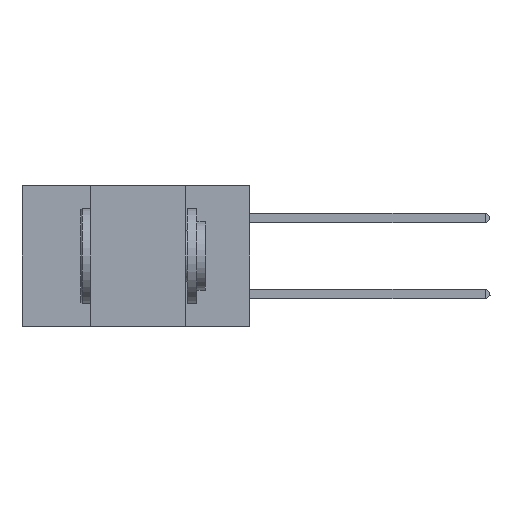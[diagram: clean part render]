
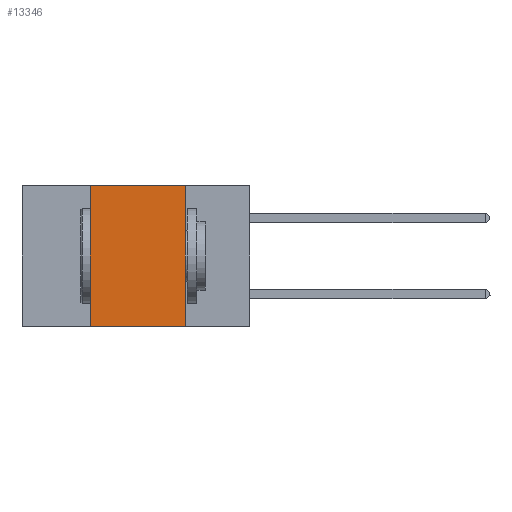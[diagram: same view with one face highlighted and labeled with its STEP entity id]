
A CAD part, left-side view. The second image highlights one B-rep face of the part: STEP entity #13346.
In plain terms, the highlighted planar face has unit normal (-1, 0, 0).
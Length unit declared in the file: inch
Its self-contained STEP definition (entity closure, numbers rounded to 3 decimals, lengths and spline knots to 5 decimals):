
#1140 = CARTESIAN_POINT ( 'NONE',  ( 0., 0.6, -0.37 ) ) ;
#1957 = DIRECTION ( 'NONE',  ( 1., 0., 0. ) ) ;
#2320 = ORIENTED_EDGE ( 'NONE', *, *, #23220, .F. ) ;
#3202 = CARTESIAN_POINT ( 'NONE',  ( 0., 0.42, 0. ) ) ;
#3345 = DIRECTION ( 'NONE',  ( 0., -1., 0. ) ) ;
#3519 = DIRECTION ( 'NONE',  ( 0., 0., -1. ) ) ;
#6569 = ORIENTED_EDGE ( 'NONE', *, *, #11300, .F. ) ;
#9484 = CARTESIAN_POINT ( 'NONE',  ( 0., 0.17, 0. ) ) ;
#9501 = VERTEX_POINT ( 'NONE', #3202 ) ;
#9570 = VECTOR ( 'NONE', #29636, 39.37008 ) ;
#9848 = FACE_OUTER_BOUND ( 'NONE', #19737, .T. ) ;
#10508 = CARTESIAN_POINT ( 'NONE',  ( 0., 0.17, -0.37 ) ) ;
#11300 = EDGE_CURVE ( 'NONE', #9501, #15618, #16460, .T. ) ;
#13346 = ADVANCED_FACE ( 'NONE', ( #9848 ), #32232, .F. ) ;
#13879 = EDGE_CURVE ( 'NONE', #15618, #23124, #34830, .T. ) ;
#14397 = CARTESIAN_POINT ( 'NONE',  ( 0., 0.6, 0. ) ) ;
#15164 = VECTOR ( 'NONE', #27417, 39.37008 ) ;
#15618 = VERTEX_POINT ( 'NONE', #9484 ) ;
#15691 = CARTESIAN_POINT ( 'NONE',  ( 0., 0.6, 0. ) ) ;
#16242 = ORIENTED_EDGE ( 'NONE', *, *, #16733, .T. ) ;
#16460 = LINE ( 'NONE', #14397, #20802 ) ;
#16482 = LINE ( 'NONE', #24002, #9570 ) ;
#16733 = EDGE_CURVE ( 'NONE', #25453, #23124, #31999, .T. ) ;
#19552 = AXIS2_PLACEMENT_3D ( 'NONE', #15691, #1957, #3519 ) ;
#19737 = EDGE_LOOP ( 'NONE', ( #23624, #6569, #2320, #16242 ) ) ;
#20802 = VECTOR ( 'NONE', #3345, 39.37008 ) ;
#21207 = CARTESIAN_POINT ( 'NONE',  ( 0., 0.42, -0.37 ) ) ;
#23124 = VERTEX_POINT ( 'NONE', #10508 ) ;
#23220 = EDGE_CURVE ( 'NONE', #25453, #9501, #16482, .T. ) ;
#23624 = ORIENTED_EDGE ( 'NONE', *, *, #13879, .F. ) ;
#24002 = CARTESIAN_POINT ( 'NONE',  ( 0., 0.42, 0. ) ) ;
#24287 = CARTESIAN_POINT ( 'NONE',  ( 0., 0.17, 0. ) ) ;
#25453 = VERTEX_POINT ( 'NONE', #21207 ) ;
#26677 = DIRECTION ( 'NONE',  ( 0., 0., -1. ) ) ;
#27417 = DIRECTION ( 'NONE',  ( 0., -1., 0. ) ) ;
#28773 = VECTOR ( 'NONE', #26677, 39.37008 ) ;
#29636 = DIRECTION ( 'NONE',  ( 0., 0., 1. ) ) ;
#31999 = LINE ( 'NONE', #1140, #15164 ) ;
#32232 = PLANE ( 'NONE',  #19552 ) ;
#34830 = LINE ( 'NONE', #24287, #28773 ) ;
